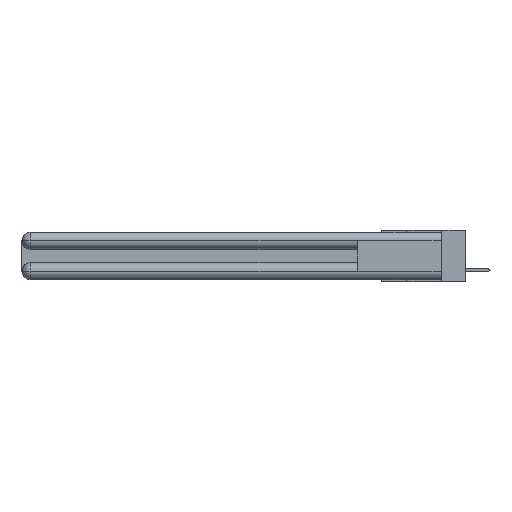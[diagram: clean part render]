
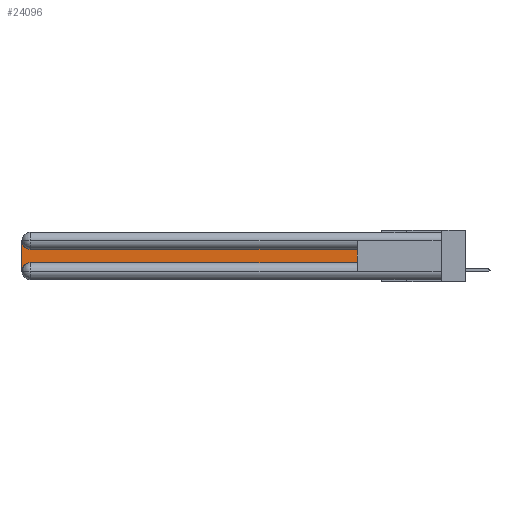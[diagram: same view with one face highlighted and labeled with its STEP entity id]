
A CAD part, left-side view. The second image highlights one B-rep face of the part: STEP entity #24096.
In plain terms, the highlighted planar face has unit normal (-1, 0, 0).
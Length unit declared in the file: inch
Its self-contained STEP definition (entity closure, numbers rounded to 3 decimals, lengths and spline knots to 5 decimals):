
#135 = CARTESIAN_POINT ( 'NONE',  ( 0.075, 2.94, -0.1225 ) ) ;
#528 = DIRECTION ( 'NONE',  ( 1., 0., 0. ) ) ;
#738 = DIRECTION ( 'NONE',  ( 0., 1., 0. ) ) ;
#2461 = EDGE_LOOP ( 'NONE', ( #29246, #25257, #11681, #26154, #18920, #8449 ) ) ;
#2515 = LINE ( 'NONE', #10222, #5653 ) ;
#3562 = DIRECTION ( 'NONE',  ( 1., 0., 0. ) ) ;
#5317 = CIRCLE ( 'NONE', #28243, 0.06 ) ;
#5649 = EDGE_CURVE ( 'NONE', #24827, #24059, #23596, .T. ) ;
#5653 = VECTOR ( 'NONE', #30617, 39.37008 ) ;
#5879 = CARTESIAN_POINT ( 'NONE',  ( 0.075, 0.6, -0.2175 ) ) ;
#6002 = VERTEX_POINT ( 'NONE', #29020 ) ;
#6691 = FACE_OUTER_BOUND ( 'NONE', #2461, .T. ) ;
#6733 = DIRECTION ( 'NONE',  ( 1., 0., 0. ) ) ;
#7111 = DIRECTION ( 'NONE',  ( 0., -1., 0. ) ) ;
#7486 = VECTOR ( 'NONE', #738, 39.37008 ) ;
#8449 = ORIENTED_EDGE ( 'NONE', *, *, #13310, .T. ) ;
#8563 = VERTEX_POINT ( 'NONE', #135 ) ;
#9145 = CARTESIAN_POINT ( 'NONE',  ( 0.075, 0.6, -0.2175 ) ) ;
#9301 = CIRCLE ( 'NONE', #13235, 0.06 ) ;
#10222 = CARTESIAN_POINT ( 'NONE',  ( 0.075, 3., -0.2175 ) ) ;
#11681 = ORIENTED_EDGE ( 'NONE', *, *, #29696, .T. ) ;
#11776 = VERTEX_POINT ( 'NONE', #20800 ) ;
#13235 = AXIS2_PLACEMENT_3D ( 'NONE', #14176, #6733, #14065 ) ;
#13310 = EDGE_CURVE ( 'NONE', #24059, #11776, #18013, .T. ) ;
#14065 = DIRECTION ( 'NONE',  ( 0., 0., -1. ) ) ;
#14176 = CARTESIAN_POINT ( 'NONE',  ( 0.075, 2.94, -0.2775 ) ) ;
#15711 = CARTESIAN_POINT ( 'NONE',  ( 0.075, 2.94, -0.0625 ) ) ;
#16912 = VECTOR ( 'NONE', #7111, 39.37008 ) ;
#17199 = CARTESIAN_POINT ( 'NONE',  ( 0.075, 3., -0.2775 ) ) ;
#17434 = LINE ( 'NONE', #30760, #7486 ) ;
#18013 = LINE ( 'NONE', #9145, #21201 ) ;
#18618 = EDGE_CURVE ( 'NONE', #23138, #24827, #9301, .T. ) ;
#18868 = PLANE ( 'NONE',  #22895 ) ;
#18920 = ORIENTED_EDGE ( 'NONE', *, *, #5649, .T. ) ;
#19153 = CARTESIAN_POINT ( 'NONE',  ( 0.075, 2.94, -0.2175 ) ) ;
#20792 = DIRECTION ( 'NONE',  ( 0., 0., -1. ) ) ;
#20800 = CARTESIAN_POINT ( 'NONE',  ( 0.075, 0.6, -0.1225 ) ) ;
#21078 = CARTESIAN_POINT ( 'NONE',  ( 0.075, 3., -0.1225 ) ) ;
#21201 = VECTOR ( 'NONE', #31697, 39.37008 ) ;
#22895 = AXIS2_PLACEMENT_3D ( 'NONE', #21078, #3562, #29030 ) ;
#23138 = VERTEX_POINT ( 'NONE', #17199 ) ;
#23596 = LINE ( 'NONE', #32217, #16912 ) ;
#24059 = VERTEX_POINT ( 'NONE', #5879 ) ;
#24096 = ADVANCED_FACE ( 'NONE', ( #6691 ), #18868, .F. ) ;
#24827 = VERTEX_POINT ( 'NONE', #19153 ) ;
#25257 = ORIENTED_EDGE ( 'NONE', *, *, #29187, .T. ) ;
#26154 = ORIENTED_EDGE ( 'NONE', *, *, #18618, .T. ) ;
#28243 = AXIS2_PLACEMENT_3D ( 'NONE', #15711, #528, #20792 ) ;
#29020 = CARTESIAN_POINT ( 'NONE',  ( 0.075, 3., -0.0625 ) ) ;
#29030 = DIRECTION ( 'NONE',  ( 0., 0., -1. ) ) ;
#29187 = EDGE_CURVE ( 'NONE', #8563, #6002, #5317, .T. ) ;
#29246 = ORIENTED_EDGE ( 'NONE', *, *, #32549, .T. ) ;
#29696 = EDGE_CURVE ( 'NONE', #6002, #23138, #2515, .T. ) ;
#30617 = DIRECTION ( 'NONE',  ( 0., 0., -1. ) ) ;
#30760 = CARTESIAN_POINT ( 'NONE',  ( 0.075, 0.6, -0.1225 ) ) ;
#31697 = DIRECTION ( 'NONE',  ( 0., 0., 1. ) ) ;
#32217 = CARTESIAN_POINT ( 'NONE',  ( 0.075, 0.6, -0.2175 ) ) ;
#32549 = EDGE_CURVE ( 'NONE', #11776, #8563, #17434, .T. ) ;
